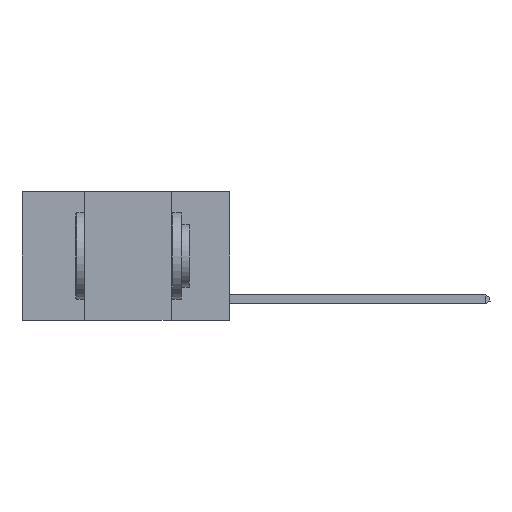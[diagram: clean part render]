
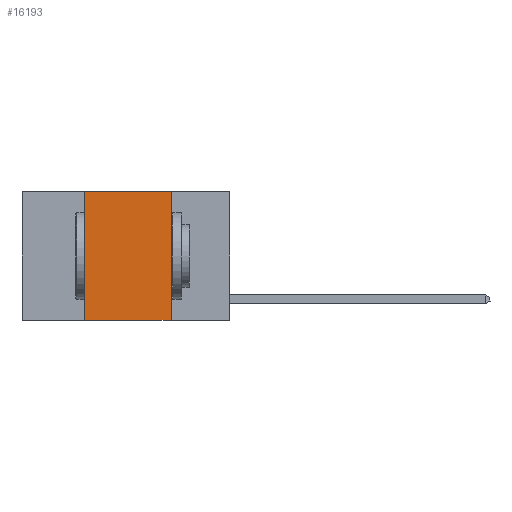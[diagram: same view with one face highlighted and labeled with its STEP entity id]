
A CAD part, left-side view. The second image highlights one B-rep face of the part: STEP entity #16193.
In plain terms, the highlighted planar face has unit normal (-1, 0, 0).
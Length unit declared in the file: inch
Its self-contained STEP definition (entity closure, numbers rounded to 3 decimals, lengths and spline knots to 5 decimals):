
#180 = DIRECTION ( 'NONE',  ( 0., 0., 1. ) ) ;
#188 = EDGE_CURVE ( 'NONE', #8883, #14762, #18951, .T. ) ;
#216 = VECTOR ( 'NONE', #15553, 39.37008 ) ;
#1309 = EDGE_CURVE ( 'NONE', #8883, #1418, #3560, .T. ) ;
#1418 = VERTEX_POINT ( 'NONE', #4082 ) ;
#1505 = VECTOR ( 'NONE', #19367, 39.37008 ) ;
#3313 = FACE_OUTER_BOUND ( 'NONE', #7607, .T. ) ;
#3421 = PLANE ( 'NONE',  #9303 ) ;
#3560 = LINE ( 'NONE', #12923, #6545 ) ;
#4082 = CARTESIAN_POINT ( 'NONE',  ( 0., 0.42, 0. ) ) ;
#4800 = CARTESIAN_POINT ( 'NONE',  ( 0., 0.17, -0.37 ) ) ;
#5008 = CARTESIAN_POINT ( 'NONE',  ( 0., 0.17, 0. ) ) ;
#5258 = EDGE_CURVE ( 'NONE', #1418, #5403, #17913, .T. ) ;
#5403 = VERTEX_POINT ( 'NONE', #5760 ) ;
#5760 = CARTESIAN_POINT ( 'NONE',  ( 0., 0.17, 0. ) ) ;
#6545 = VECTOR ( 'NONE', #180, 39.37008 ) ;
#7607 = EDGE_LOOP ( 'NONE', ( #12184, #16426, #16264, #14289 ) ) ;
#8883 = VERTEX_POINT ( 'NONE', #18586 ) ;
#9303 = AXIS2_PLACEMENT_3D ( 'NONE', #14372, #9599, #14676 ) ;
#9599 = DIRECTION ( 'NONE',  ( 1., 0., 0. ) ) ;
#9800 = VECTOR ( 'NONE', #10558, 39.37008 ) ;
#9903 = LINE ( 'NONE', #5008, #1505 ) ;
#10558 = DIRECTION ( 'NONE',  ( 0., -1., 0. ) ) ;
#11444 = CARTESIAN_POINT ( 'NONE',  ( 0., 0.6, 0. ) ) ;
#12184 = ORIENTED_EDGE ( 'NONE', *, *, #16216, .F. ) ;
#12923 = CARTESIAN_POINT ( 'NONE',  ( 0., 0.42, 0. ) ) ;
#14166 = CARTESIAN_POINT ( 'NONE',  ( 0., 0.6, -0.37 ) ) ;
#14289 = ORIENTED_EDGE ( 'NONE', *, *, #188, .T. ) ;
#14372 = CARTESIAN_POINT ( 'NONE',  ( 0., 0.6, 0. ) ) ;
#14676 = DIRECTION ( 'NONE',  ( 0., 0., -1. ) ) ;
#14762 = VERTEX_POINT ( 'NONE', #4800 ) ;
#15553 = DIRECTION ( 'NONE',  ( 0., -1., 0. ) ) ;
#16193 = ADVANCED_FACE ( 'NONE', ( #3313 ), #3421, .F. ) ;
#16216 = EDGE_CURVE ( 'NONE', #5403, #14762, #9903, .T. ) ;
#16264 = ORIENTED_EDGE ( 'NONE', *, *, #1309, .F. ) ;
#16426 = ORIENTED_EDGE ( 'NONE', *, *, #5258, .F. ) ;
#17913 = LINE ( 'NONE', #11444, #9800 ) ;
#18586 = CARTESIAN_POINT ( 'NONE',  ( 0., 0.42, -0.37 ) ) ;
#18951 = LINE ( 'NONE', #14166, #216 ) ;
#19367 = DIRECTION ( 'NONE',  ( 0., 0., -1. ) ) ;
